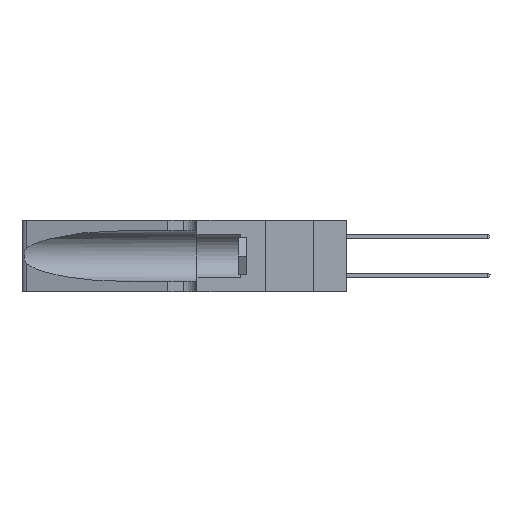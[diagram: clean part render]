
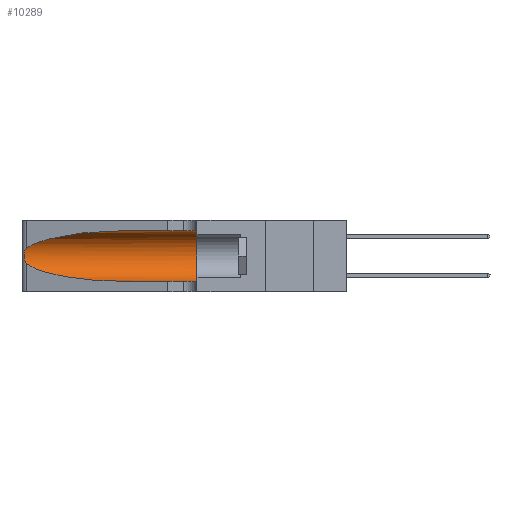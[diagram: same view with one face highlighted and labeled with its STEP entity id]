
A CAD part, left-side view. The second image highlights one B-rep face of the part: STEP entity #10289.
In plain terms, the highlighted cylindrical face has radius 3.308 mm (diameter 6.617 mm), a partial arc.
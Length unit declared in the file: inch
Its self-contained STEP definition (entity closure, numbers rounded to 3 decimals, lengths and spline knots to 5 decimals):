
#590 = ORIENTED_EDGE ( 'NONE', *, *, #16124, .T. ) ;
#925 = CYLINDRICAL_SURFACE ( 'NONE', #17526, 0.13025 ) ;
#1751 = CARTESIAN_POINT ( 'NONE',  ( 0.25856, 1.23593, 0.16098 ) ) ;
#1870 = CARTESIAN_POINT ( 'NONE',  ( 0.26075, 1.23896, 0.19203 ) ) ;
#2093 = CARTESIAN_POINT ( 'NONE',  ( 0.25487, 1.22718, 0.22369 ) ) ;
#2219 = CARTESIAN_POINT ( 'NONE',  ( 0.26075, 1.23896, 0.178 ) ) ;
#2253 = CARTESIAN_POINT ( 'NONE',  ( 0.25487, 1.22718, 0.14631 ) ) ;
#2291 = ORIENTED_EDGE ( 'NONE', *, *, #13063, .T. ) ;
#3703 = AXIS2_PLACEMENT_3D ( 'NONE', #7464, #27451, #21886 ) ;
#4453 = CARTESIAN_POINT ( 'NONE',  ( 0.1305, 1.61858, 0.05475 ) ) ;
#4677 = CARTESIAN_POINT ( 'NONE',  ( 0.25787, 1.23484, 0.2124 ) ) ;
#5223 = CARTESIAN_POINT ( 'NONE',  ( 0.1305, 0.72297, 0.31525 ) ) ;
#5364 = VERTEX_POINT ( 'NONE', #18611 ) ;
#6961 =( BOUNDED_CURVE ( )  B_SPLINE_CURVE ( 3, ( #2253, #7927, #27690, #36347 ),
 .UNSPECIFIED., .F., .F. ) 
 B_SPLINE_CURVE_WITH_KNOTS ( ( 4, 4 ),
 ( 3.44316, 4.71239 ),
 .UNSPECIFIED. ) 
 CURVE ( )  GEOMETRIC_REPRESENTATION_ITEM ( )  RATIONAL_B_SPLINE_CURVE ( ( 1., 0.87, 0.87, 1. ) ) 
 REPRESENTATION_ITEM ( '' )  );
#7187 = DIRECTION ( 'NONE',  ( 0., -1., 0. ) ) ;
#7442 = VECTOR ( 'NONE', #7187, 39.37008 ) ;
#7464 = CARTESIAN_POINT ( 'NONE',  ( 0.1305, 0.35, 0.185 ) ) ;
#7927 = CARTESIAN_POINT ( 'NONE',  ( 0.2373, 1.15595, 0.08982 ) ) ;
#8139 = CARTESIAN_POINT ( 'NONE',  ( 0.1305, 0.35, 0.05475 ) ) ;
#9116 = VERTEX_POINT ( 'NONE', #8139 ) ;
#9208 = B_SPLINE_CURVE_WITH_KNOTS ( 'NONE', 3,
 ( #2093, #35716, #27646, #4677, #10733, #30147, #1870, #2219, #35603, #1751, #24671, #24555, #21848, #13440 ),
 .UNSPECIFIED., .F., .F.,
 ( 4, 2, 2, 2, 2, 2, 4 ),
 ( 0., 0.00027, 0.00053, 0.00107, 0.0016, 0.00187, 0.00214 ),
 .UNSPECIFIED. ) ;
#10289 = ADVANCED_FACE ( 'NONE', ( #26537 ), #925, .F. ) ;
#10310 = CARTESIAN_POINT ( 'NONE',  ( 0.1305, 1.61858, 0.185 ) ) ;
#10596 = LINE ( 'NONE', #29706, #26991 ) ;
#10733 = CARTESIAN_POINT ( 'NONE',  ( 0.25854, 1.2359, 0.20912 ) ) ;
#12841 = CARTESIAN_POINT ( 'NONE',  ( 0.25487, 1.22718, 0.22369 ) ) ;
#13063 = EDGE_CURVE ( 'NONE', #18838, #5364, #25503, .T. ) ;
#13440 = CARTESIAN_POINT ( 'NONE',  ( 0.25487, 1.22718, 0.14631 ) ) ;
#13582 = CARTESIAN_POINT ( 'NONE',  ( 0.25487, 1.22718, 0.14631 ) ) ;
#13640 = ORIENTED_EDGE ( 'NONE', *, *, #23314, .T. ) ;
#15988 = DIRECTION ( 'NONE',  ( 0., 0., -1. ) ) ;
#16124 = EDGE_CURVE ( 'NONE', #31500, #31018, #6961, .T. ) ;
#17526 = AXIS2_PLACEMENT_3D ( 'NONE', #10310, #32948, #15988 ) ;
#18611 = CARTESIAN_POINT ( 'NONE',  ( 0.25487, 1.22718, 0.22369 ) ) ;
#18838 = VERTEX_POINT ( 'NONE', #5223 ) ;
#21104 = CARTESIAN_POINT ( 'NONE',  ( 0.2373, 1.15595, 0.28018 ) ) ;
#21231 = CARTESIAN_POINT ( 'NONE',  ( 0.1305, 0.72297, 0.31525 ) ) ;
#21848 = CARTESIAN_POINT ( 'NONE',  ( 0.25555, 1.22993, 0.14849 ) ) ;
#21886 = DIRECTION ( 'NONE',  ( 0., 0., 1. ) ) ;
#22466 = ORIENTED_EDGE ( 'NONE', *, *, #36004, .T. ) ;
#22742 = CARTESIAN_POINT ( 'NONE',  ( 0.1305, 0.72297, 0.05475 ) ) ;
#23314 = EDGE_CURVE ( 'NONE', #5364, #31500, #9208, .T. ) ;
#23319 = ORIENTED_EDGE ( 'NONE', *, *, #26574, .F. ) ;
#23888 = DIRECTION ( 'NONE',  ( 0., -1., 0. ) ) ;
#24555 = CARTESIAN_POINT ( 'NONE',  ( 0.25639, 1.23186, 0.15144 ) ) ;
#24671 = CARTESIAN_POINT ( 'NONE',  ( 0.25789, 1.23486, 0.15765 ) ) ;
#25503 =( BOUNDED_CURVE ( )  B_SPLINE_CURVE ( 3, ( #21231, #35223, #21104, #12841 ),
 .UNSPECIFIED., .F., .F. ) 
 B_SPLINE_CURVE_WITH_KNOTS ( ( 4, 4 ),
 ( 1.5708, 2.84003 ),
 .UNSPECIFIED. ) 
 CURVE ( )  GEOMETRIC_REPRESENTATION_ITEM ( )  RATIONAL_B_SPLINE_CURVE ( ( 1., 0.87, 0.87, 1. ) ) 
 REPRESENTATION_ITEM ( '' )  );
#26471 = EDGE_CURVE ( 'NONE', #18838, #36369, #10596, .T. ) ;
#26537 = FACE_OUTER_BOUND ( 'NONE', #30510, .T. ) ;
#26574 = EDGE_CURVE ( 'NONE', #36369, #9116, #35832, .T. ) ;
#26991 = VECTOR ( 'NONE', #23888, 39.37008 ) ;
#27451 = DIRECTION ( 'NONE',  ( 0., 1., 0. ) ) ;
#27646 = CARTESIAN_POINT ( 'NONE',  ( 0.25639, 1.23184, 0.21858 ) ) ;
#27690 = CARTESIAN_POINT ( 'NONE',  ( 0.18966, 0.96281, 0.05475 ) ) ;
#28192 = LINE ( 'NONE', #4453, #7442 ) ;
#28771 = CARTESIAN_POINT ( 'NONE',  ( 0.1305, 0.35, 0.31525 ) ) ;
#29706 = CARTESIAN_POINT ( 'NONE',  ( 0.1305, 1.61858, 0.31525 ) ) ;
#30147 = CARTESIAN_POINT ( 'NONE',  ( 0.26018, 1.23835, 0.19895 ) ) ;
#30510 = EDGE_LOOP ( 'NONE', ( #2291, #13640, #590, #22466, #23319, #33032 ) ) ;
#31018 = VERTEX_POINT ( 'NONE', #22742 ) ;
#31500 = VERTEX_POINT ( 'NONE', #13582 ) ;
#32948 = DIRECTION ( 'NONE',  ( 0., -1., 0. ) ) ;
#33032 = ORIENTED_EDGE ( 'NONE', *, *, #26471, .F. ) ;
#35223 = CARTESIAN_POINT ( 'NONE',  ( 0.18966, 0.96281, 0.31525 ) ) ;
#35603 = CARTESIAN_POINT ( 'NONE',  ( 0.26017, 1.23833, 0.17102 ) ) ;
#35716 = CARTESIAN_POINT ( 'NONE',  ( 0.25555, 1.22994, 0.2215 ) ) ;
#35832 = CIRCLE ( 'NONE', #3703, 0.13025 ) ;
#36004 = EDGE_CURVE ( 'NONE', #31018, #9116, #28192, .T. ) ;
#36347 = CARTESIAN_POINT ( 'NONE',  ( 0.1305, 0.72297, 0.05475 ) ) ;
#36369 = VERTEX_POINT ( 'NONE', #28771 ) ;
